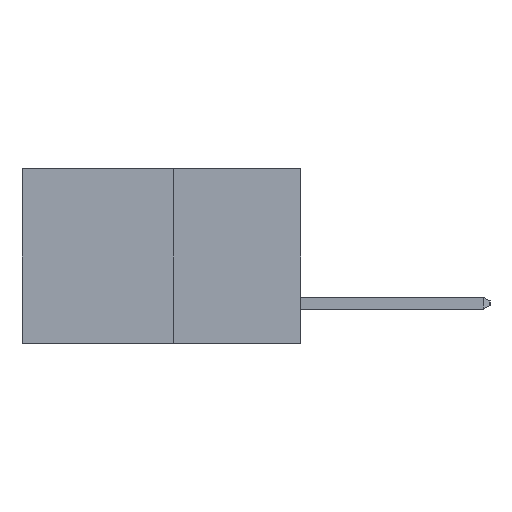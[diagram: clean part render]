
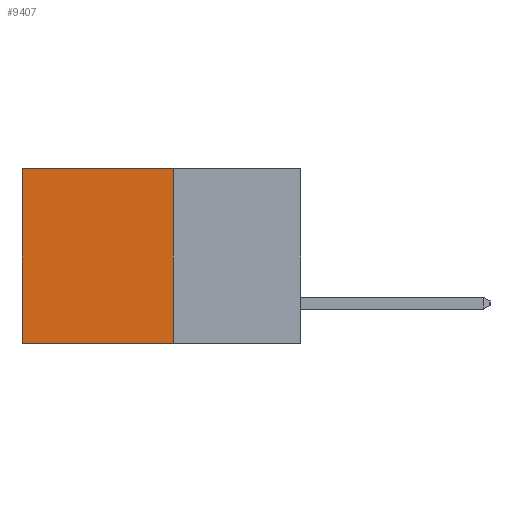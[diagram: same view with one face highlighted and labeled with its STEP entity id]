
A CAD part, left-side view. The second image highlights one B-rep face of the part: STEP entity #9407.
In plain terms, the highlighted planar face has unit normal (-1, 0, 0).
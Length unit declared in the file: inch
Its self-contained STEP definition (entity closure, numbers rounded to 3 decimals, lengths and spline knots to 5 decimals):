
#259 = DIRECTION ( 'NONE',  ( 0., 0., -1. ) ) ;
#312 = CARTESIAN_POINT ( 'NONE',  ( 0.277, 0.59, 0. ) ) ;
#319 = VERTEX_POINT ( 'NONE', #312 ) ;
#338 = CARTESIAN_POINT ( 'NONE',  ( 0.277, 0.59, -0.37 ) ) ;
#842 = VERTEX_POINT ( 'NONE', #9306 ) ;
#1028 = LINE ( 'NONE', #338, #10011 ) ;
#1992 = VECTOR ( 'NONE', #4620, 39.37008 ) ;
#2313 = VERTEX_POINT ( 'NONE', #2566 ) ;
#2566 = CARTESIAN_POINT ( 'NONE',  ( 0.277, 0.27, 0. ) ) ;
#2921 = ORIENTED_EDGE ( 'NONE', *, *, #10018, .F. ) ;
#3785 = FACE_OUTER_BOUND ( 'NONE', #6462, .T. ) ;
#3788 = LINE ( 'NONE', #7724, #10855 ) ;
#4364 = LINE ( 'NONE', #4882, #1992 ) ;
#4600 = ORIENTED_EDGE ( 'NONE', *, *, #6249, .F. ) ;
#4620 = DIRECTION ( 'NONE',  ( 0., 1., 0. ) ) ;
#4838 = CARTESIAN_POINT ( 'NONE',  ( 0.277, 0.59, -0.37 ) ) ;
#4882 = CARTESIAN_POINT ( 'NONE',  ( 0.277, 0.27, 0. ) ) ;
#5209 = DIRECTION ( 'NONE',  ( 0., 0., -1. ) ) ;
#5408 = CARTESIAN_POINT ( 'NONE',  ( 0.277, 0.27, -0.37 ) ) ;
#5467 = ORIENTED_EDGE ( 'NONE', *, *, #8488, .T. ) ;
#5574 = AXIS2_PLACEMENT_3D ( 'NONE', #7407, #8355, #8357 ) ;
#6249 = EDGE_CURVE ( 'NONE', #2313, #842, #9807, .T. ) ;
#6462 = EDGE_LOOP ( 'NONE', ( #8773, #2921, #4600, #5467 ) ) ;
#7399 = PLANE ( 'NONE',  #5574 ) ;
#7407 = CARTESIAN_POINT ( 'NONE',  ( 0.277, 0.27, -0.37 ) ) ;
#7527 = VECTOR ( 'NONE', #5209, 39.37008 ) ;
#7570 = DIRECTION ( 'NONE',  ( 0., 1., 0. ) ) ;
#7724 = CARTESIAN_POINT ( 'NONE',  ( 0.277, 0.27, -0.37 ) ) ;
#7914 = EDGE_CURVE ( 'NONE', #319, #9475, #1028, .T. ) ;
#8355 = DIRECTION ( 'NONE',  ( 1., 0., 0. ) ) ;
#8357 = DIRECTION ( 'NONE',  ( 0., 0., -1. ) ) ;
#8488 = EDGE_CURVE ( 'NONE', #2313, #319, #4364, .T. ) ;
#8773 = ORIENTED_EDGE ( 'NONE', *, *, #7914, .T. ) ;
#9306 = CARTESIAN_POINT ( 'NONE',  ( 0.277, 0.27, -0.37 ) ) ;
#9407 = ADVANCED_FACE ( 'NONE', ( #3785 ), #7399, .F. ) ;
#9475 = VERTEX_POINT ( 'NONE', #4838 ) ;
#9807 = LINE ( 'NONE', #5408, #7527 ) ;
#10011 = VECTOR ( 'NONE', #259, 39.37008 ) ;
#10018 = EDGE_CURVE ( 'NONE', #842, #9475, #3788, .T. ) ;
#10855 = VECTOR ( 'NONE', #7570, 39.37008 ) ;
